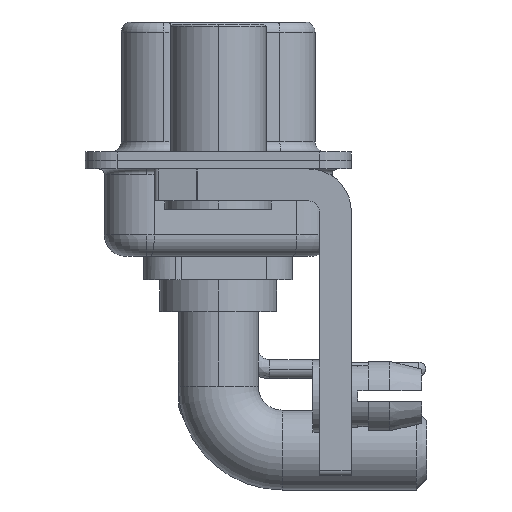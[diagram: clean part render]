
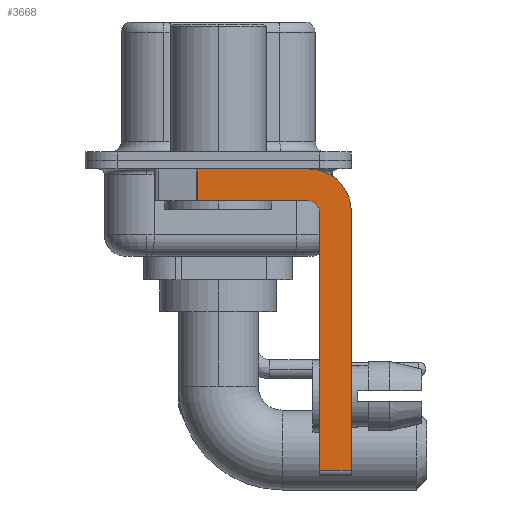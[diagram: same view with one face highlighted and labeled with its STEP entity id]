
A CAD part, left-side view. The second image highlights one B-rep face of the part: STEP entity #3668.
In plain terms, the highlighted planar face has unit normal (-1, 0, 0).
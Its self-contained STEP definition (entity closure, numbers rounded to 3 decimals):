
#157 = LINE ( 'NONE', #15583, #11148 ) ;
#1084 = CARTESIAN_POINT ( 'NONE',  ( -2.9, -4.75, -14.55 ) ) ;
#1262 = EDGE_LOOP ( 'NONE', ( #4952, #18211, #2388, #16539, #17402, #11036, #2595, #6402 ) ) ;
#1458 = DIRECTION ( 'NONE',  ( 0., 0., -1. ) ) ;
#1687 = CIRCLE ( 'NONE', #9305, 2. ) ;
#2388 = ORIENTED_EDGE ( 'NONE', *, *, #2431, .F. ) ;
#2431 = EDGE_CURVE ( 'NONE', #22559, #7675, #10985, .T. ) ;
#2595 = ORIENTED_EDGE ( 'NONE', *, *, #14813, .F. ) ;
#3164 = FACE_OUTER_BOUND ( 'NONE', #1262, .T. ) ;
#3304 = DIRECTION ( 'NONE',  ( -1., 0., 0. ) ) ;
#3668 = ADVANCED_FACE ( 'NONE', ( #3164 ), #26990, .F. ) ;
#4175 = CARTESIAN_POINT ( 'NONE',  ( -2.9, -4.25, -0.4 ) ) ;
#4224 = DIRECTION ( 'NONE',  ( 1., 0., 0. ) ) ;
#4850 = CARTESIAN_POINT ( 'NONE',  ( -2.9, 0.978, -0.4 ) ) ;
#4949 = EDGE_CURVE ( 'NONE', #16253, #22559, #21809, .T. ) ;
#4952 = ORIENTED_EDGE ( 'NONE', *, *, #12694, .F. ) ;
#5218 = CARTESIAN_POINT ( 'NONE',  ( -2.9, -6.25, -14.55 ) ) ;
#5299 = DIRECTION ( 'NONE',  ( 0., 0., -1. ) ) ;
#5669 = CARTESIAN_POINT ( 'NONE',  ( -2.9, 3., -0.4 ) ) ;
#6123 = AXIS2_PLACEMENT_3D ( 'NONE', #13980, #7789, #22920 ) ;
#6402 = ORIENTED_EDGE ( 'NONE', *, *, #22362, .F. ) ;
#6450 = LINE ( 'NONE', #7264, #16044 ) ;
#6761 = EDGE_CURVE ( 'NONE', #11025, #7675, #6450, .T. ) ;
#7264 = CARTESIAN_POINT ( 'NONE',  ( -2.9, 0.978, -1.9 ) ) ;
#7651 = CARTESIAN_POINT ( 'NONE',  ( -2.9, -6.25, -2.4 ) ) ;
#7675 = VERTEX_POINT ( 'NONE', #17817 ) ;
#7789 = DIRECTION ( 'NONE',  ( 1., 0., 0. ) ) ;
#8526 = CARTESIAN_POINT ( 'NONE',  ( -2.9, -4.75, -2.4 ) ) ;
#9076 = VERTEX_POINT ( 'NONE', #9404 ) ;
#9305 = AXIS2_PLACEMENT_3D ( 'NONE', #14622, #4224, #25676 ) ;
#9404 = CARTESIAN_POINT ( 'NONE',  ( -2.9, -6.25, -2.4 ) ) ;
#9532 = VECTOR ( 'NONE', #23055, 1000. ) ;
#9565 = VECTOR ( 'NONE', #1458, 1000. ) ;
#10985 = LINE ( 'NONE', #17281, #23734 ) ;
#11025 = VERTEX_POINT ( 'NONE', #4850 ) ;
#11036 = ORIENTED_EDGE ( 'NONE', *, *, #22596, .T. ) ;
#11148 = VECTOR ( 'NONE', #15176, 1000. ) ;
#12292 = DIRECTION ( 'NONE',  ( 0., -1., 0. ) ) ;
#12301 = CARTESIAN_POINT ( 'NONE',  ( -2.9, -4.25, -2.4 ) ) ;
#12694 = EDGE_CURVE ( 'NONE', #11025, #17702, #22917, .T. ) ;
#12769 = EDGE_CURVE ( 'NONE', #27387, #16253, #16341, .T. ) ;
#13980 = CARTESIAN_POINT ( 'NONE',  ( -2.9, -4.25, -2.4 ) ) ;
#14622 = CARTESIAN_POINT ( 'NONE',  ( -2.9, -4.25, -2.4 ) ) ;
#14813 = EDGE_CURVE ( 'NONE', #9076, #22281, #26480, .T. ) ;
#15176 = DIRECTION ( 'NONE',  ( 0., -1., 0. ) ) ;
#15583 = CARTESIAN_POINT ( 'NONE',  ( -2.9, -4.25, -14.55 ) ) ;
#16044 = VECTOR ( 'NONE', #5299, 1000. ) ;
#16253 = VERTEX_POINT ( 'NONE', #8526 ) ;
#16341 = LINE ( 'NONE', #16612, #9532 ) ;
#16539 = ORIENTED_EDGE ( 'NONE', *, *, #4949, .F. ) ;
#16612 = CARTESIAN_POINT ( 'NONE',  ( -2.9, -4.75, -14.8 ) ) ;
#17281 = CARTESIAN_POINT ( 'NONE',  ( -2.9, -4.25, -1.9 ) ) ;
#17402 = ORIENTED_EDGE ( 'NONE', *, *, #12769, .F. ) ;
#17702 = VERTEX_POINT ( 'NONE', #4175 ) ;
#17817 = CARTESIAN_POINT ( 'NONE',  ( -2.9, 0.978, -1.9 ) ) ;
#18211 = ORIENTED_EDGE ( 'NONE', *, *, #6761, .T. ) ;
#20689 = DIRECTION ( 'NONE',  ( 0., 0., 1. ) ) ;
#21613 = CARTESIAN_POINT ( 'NONE',  ( -2.9, -4.25, -1.9 ) ) ;
#21809 = CIRCLE ( 'NONE', #22266, 0.5 ) ;
#22266 = AXIS2_PLACEMENT_3D ( 'NONE', #12301, #3304, #20689 ) ;
#22281 = VERTEX_POINT ( 'NONE', #5218 ) ;
#22362 = EDGE_CURVE ( 'NONE', #17702, #9076, #1687, .T. ) ;
#22559 = VERTEX_POINT ( 'NONE', #21613 ) ;
#22596 = EDGE_CURVE ( 'NONE', #27387, #22281, #157, .T. ) ;
#22917 = LINE ( 'NONE', #5669, #25649 ) ;
#22920 = DIRECTION ( 'NONE',  ( 0., 0., -1. ) ) ;
#23055 = DIRECTION ( 'NONE',  ( 0., 0., 1. ) ) ;
#23317 = DIRECTION ( 'NONE',  ( 0., 1., 0. ) ) ;
#23734 = VECTOR ( 'NONE', #23317, 1000. ) ;
#25649 = VECTOR ( 'NONE', #12292, 1000. ) ;
#25676 = DIRECTION ( 'NONE',  ( 0., 0., -1. ) ) ;
#26480 = LINE ( 'NONE', #7651, #9565 ) ;
#26990 = PLANE ( 'NONE',  #6123 ) ;
#27387 = VERTEX_POINT ( 'NONE', #1084 ) ;
